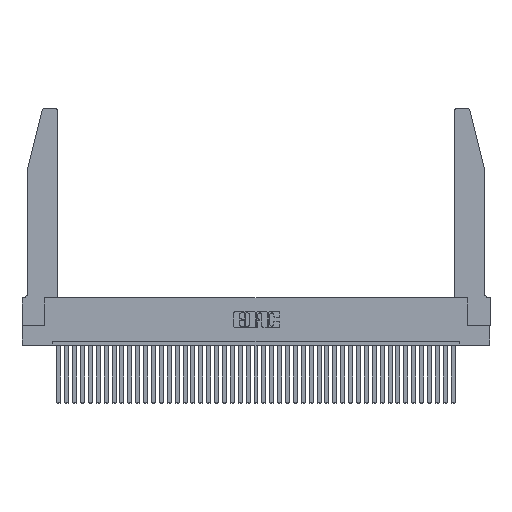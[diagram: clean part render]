
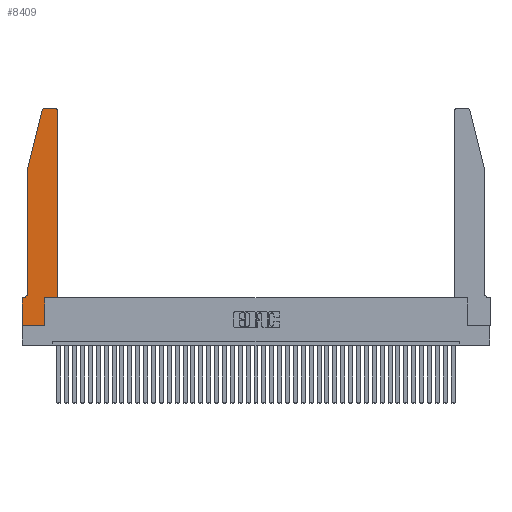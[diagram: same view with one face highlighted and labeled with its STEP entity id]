
A CAD part, top view. The second image highlights one B-rep face of the part: STEP entity #8409.
In plain terms, the highlighted planar face has unit normal (0, 0, 1).
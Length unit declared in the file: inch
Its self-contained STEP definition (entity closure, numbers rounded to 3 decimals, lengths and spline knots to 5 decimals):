
#886 = ORIENTED_EDGE ( 'NONE', *, *, #18709, .T. ) ;
#936 = DIRECTION ( 'NONE',  ( 1., 0., 0. ) ) ;
#979 = VERTEX_POINT ( 'NONE', #22835 ) ;
#1300 = CARTESIAN_POINT ( 'NONE',  ( 0.2865, 0., 0.37 ) ) ;
#1639 = VERTEX_POINT ( 'NONE', #4254 ) ;
#1700 = CARTESIAN_POINT ( 'NONE',  ( 0.4505, 0.35, 0.37 ) ) ;
#2292 = CARTESIAN_POINT ( 'NONE',  ( 0.2865, 0.35, 0.37 ) ) ;
#2448 = VECTOR ( 'NONE', #22228, 39.37008 ) ;
#2922 = LINE ( 'NONE', #38307, #2448 ) ;
#2924 = CARTESIAN_POINT ( 'NONE',  ( 0., 0.35, 0.37 ) ) ;
#3045 = LINE ( 'NONE', #5219, #31289 ) ;
#3803 = LINE ( 'NONE', #17365, #31007 ) ;
#4254 = CARTESIAN_POINT ( 'NONE',  ( 0.0755, 0.42, 0.37 ) ) ;
#4364 = DIRECTION ( 'NONE',  ( 0., 1., 0. ) ) ;
#4440 = LINE ( 'NONE', #9946, #17579 ) ;
#4630 = ORIENTED_EDGE ( 'NONE', *, *, #14583, .T. ) ;
#4757 = DIRECTION ( 'NONE',  ( -1., 0., 0. ) ) ;
#4987 = ORIENTED_EDGE ( 'NONE', *, *, #40740, .T. ) ;
#5219 = CARTESIAN_POINT ( 'NONE',  ( 0., 0., 0.37 ) ) ;
#5370 = ORIENTED_EDGE ( 'NONE', *, *, #9482, .T. ) ;
#6107 = VERTEX_POINT ( 'NONE', #1700 ) ;
#6317 = EDGE_CURVE ( 'NONE', #33854, #8645, #3045, .T. ) ;
#7628 = FACE_OUTER_BOUND ( 'NONE', #29899, .T. ) ;
#8078 = VERTEX_POINT ( 'NONE', #14900 ) ;
#8409 = ADVANCED_FACE ( 'NONE', ( #7628 ), #20192, .T. ) ;
#8547 = VERTEX_POINT ( 'NONE', #27357 ) ;
#8645 = VERTEX_POINT ( 'NONE', #1300 ) ;
#9482 = EDGE_CURVE ( 'NONE', #8078, #20323, #23128, .T. ) ;
#9830 = CARTESIAN_POINT ( 'NONE',  ( 0.4205, 2.72, 0.37 ) ) ;
#9946 = CARTESIAN_POINT ( 'NONE',  ( 0.0755, 2., 0.37 ) ) ;
#10032 = VECTOR ( 'NONE', #19078, 39.37008 ) ;
#12411 = ORIENTED_EDGE ( 'NONE', *, *, #6317, .T. ) ;
#13214 = DIRECTION ( 'NONE',  ( 0., -1., 0. ) ) ;
#13339 = ORIENTED_EDGE ( 'NONE', *, *, #22632, .T. ) ;
#14583 = EDGE_CURVE ( 'NONE', #21754, #6107, #18103, .T. ) ;
#14900 = CARTESIAN_POINT ( 'NONE',  ( 0.4505, 2.72, 0.37 ) ) ;
#15164 = EDGE_CURVE ( 'NONE', #6107, #8078, #3803, .T. ) ;
#15720 = DIRECTION ( 'NONE',  ( 0., 0., -1. ) ) ;
#15925 = LINE ( 'NONE', #33526, #38588 ) ;
#16945 = LINE ( 'NONE', #40522, #32047 ) ;
#17365 = CARTESIAN_POINT ( 'NONE',  ( 0.4505, 0.35, 0.37 ) ) ;
#17579 = VECTOR ( 'NONE', #13214, 39.37008 ) ;
#18103 = LINE ( 'NONE', #33170, #41753 ) ;
#18487 = DIRECTION ( 'NONE',  ( 1., 0., 0. ) ) ;
#18709 = EDGE_CURVE ( 'NONE', #38470, #22651, #15925, .T. ) ;
#19078 = DIRECTION ( 'NONE',  ( 0., 1., 0. ) ) ;
#19919 = AXIS2_PLACEMENT_3D ( 'NONE', #39764, #30049, #20471 ) ;
#20192 = PLANE ( 'NONE',  #19919 ) ;
#20323 = VERTEX_POINT ( 'NONE', #23372 ) ;
#20471 = DIRECTION ( 'NONE',  ( 1., 0., 0. ) ) ;
#20764 = CIRCLE ( 'NONE', #25898, 0.03 ) ;
#21022 = CARTESIAN_POINT ( 'NONE',  ( 0.0755, 2., 0.37 ) ) ;
#21620 = LINE ( 'NONE', #29491, #10032 ) ;
#21754 = VERTEX_POINT ( 'NONE', #2292 ) ;
#22228 = DIRECTION ( 'NONE',  ( -1., 0., 0. ) ) ;
#22533 = CARTESIAN_POINT ( 'NONE',  ( 0.0055, 0.35, 0.37 ) ) ;
#22632 = EDGE_CURVE ( 'NONE', #20323, #979, #2922, .T. ) ;
#22651 = VERTEX_POINT ( 'NONE', #2924 ) ;
#22835 = CARTESIAN_POINT ( 'NONE',  ( 0.284, 2.75, 0.37 ) ) ;
#23128 = CIRCLE ( 'NONE', #28299, 0.03 ) ;
#23372 = CARTESIAN_POINT ( 'NONE',  ( 0.4205, 2.75, 0.37 ) ) ;
#23572 = DIRECTION ( 'NONE',  ( 1., 0., 0. ) ) ;
#23609 = CARTESIAN_POINT ( 'NONE',  ( 0.284, 2.72, 0.37 ) ) ;
#24144 = LINE ( 'NONE', #34966, #27170 ) ;
#24905 = EDGE_CURVE ( 'NONE', #979, #8547, #20764, .T. ) ;
#25219 = AXIS2_PLACEMENT_3D ( 'NONE', #37968, #15720, #37676 ) ;
#25409 = ORIENTED_EDGE ( 'NONE', *, *, #24905, .T. ) ;
#25898 = AXIS2_PLACEMENT_3D ( 'NONE', #23609, #33618, #936 ) ;
#26341 = ORIENTED_EDGE ( 'NONE', *, *, #31799, .T. ) ;
#27170 = VECTOR ( 'NONE', #35099, 39.37008 ) ;
#27357 = CARTESIAN_POINT ( 'NONE',  ( 0.25487, 2.72718, 0.37 ) ) ;
#27564 = DIRECTION ( 'NONE',  ( 0., -1., 0. ) ) ;
#27802 = EDGE_CURVE ( 'NONE', #36240, #1639, #4440, .T. ) ;
#28231 = ORIENTED_EDGE ( 'NONE', *, *, #27802, .T. ) ;
#28299 = AXIS2_PLACEMENT_3D ( 'NONE', #9830, #35633, #29404 ) ;
#28926 = CARTESIAN_POINT ( 'NONE',  ( 0., 0., 0.37 ) ) ;
#29404 = DIRECTION ( 'NONE',  ( 1., 0., 0. ) ) ;
#29491 = CARTESIAN_POINT ( 'NONE',  ( 0.2865, 0.35, 0.37 ) ) ;
#29899 = EDGE_LOOP ( 'NONE', ( #13339, #25409, #26341, #28231, #4987, #886, #33813, #12411, #41584, #4630, #33203, #5370 ) ) ;
#30049 = DIRECTION ( 'NONE',  ( 0., 0., 1. ) ) ;
#31007 = VECTOR ( 'NONE', #4364, 39.37008 ) ;
#31289 = VECTOR ( 'NONE', #18487, 39.37008 ) ;
#31799 = EDGE_CURVE ( 'NONE', #8547, #36240, #24144, .T. ) ;
#32047 = VECTOR ( 'NONE', #27564, 39.37008 ) ;
#33170 = CARTESIAN_POINT ( 'NONE',  ( 0.4505, 0.35, 0.37 ) ) ;
#33203 = ORIENTED_EDGE ( 'NONE', *, *, #15164, .T. ) ;
#33495 = CIRCLE ( 'NONE', #25219, 0.07 ) ;
#33526 = CARTESIAN_POINT ( 'NONE',  ( 0.0755, 0.35, 0.37 ) ) ;
#33618 = DIRECTION ( 'NONE',  ( 0., 0., 1. ) ) ;
#33813 = ORIENTED_EDGE ( 'NONE', *, *, #40067, .T. ) ;
#33854 = VERTEX_POINT ( 'NONE', #28926 ) ;
#34966 = CARTESIAN_POINT ( 'NONE',  ( 0.0755, 2., 0.37 ) ) ;
#35099 = DIRECTION ( 'NONE',  ( -0.239, -0.971, 0. ) ) ;
#35633 = DIRECTION ( 'NONE',  ( 0., 0., 1. ) ) ;
#36240 = VERTEX_POINT ( 'NONE', #21022 ) ;
#37676 = DIRECTION ( 'NONE',  ( -1., 0., 0. ) ) ;
#37892 = EDGE_CURVE ( 'NONE', #8645, #21754, #21620, .T. ) ;
#37968 = CARTESIAN_POINT ( 'NONE',  ( 0.0055, 0.42, 0.37 ) ) ;
#38307 = CARTESIAN_POINT ( 'NONE',  ( 0.2605, 2.75, 0.37 ) ) ;
#38470 = VERTEX_POINT ( 'NONE', #22533 ) ;
#38588 = VECTOR ( 'NONE', #4757, 39.37008 ) ;
#39764 = CARTESIAN_POINT ( 'NONE',  ( 0., 0.35, 0.37 ) ) ;
#40067 = EDGE_CURVE ( 'NONE', #22651, #33854, #16945, .T. ) ;
#40522 = CARTESIAN_POINT ( 'NONE',  ( 0., 0., 0.37 ) ) ;
#40740 = EDGE_CURVE ( 'NONE', #1639, #38470, #33495, .T. ) ;
#41584 = ORIENTED_EDGE ( 'NONE', *, *, #37892, .T. ) ;
#41753 = VECTOR ( 'NONE', #23572, 39.37008 ) ;
